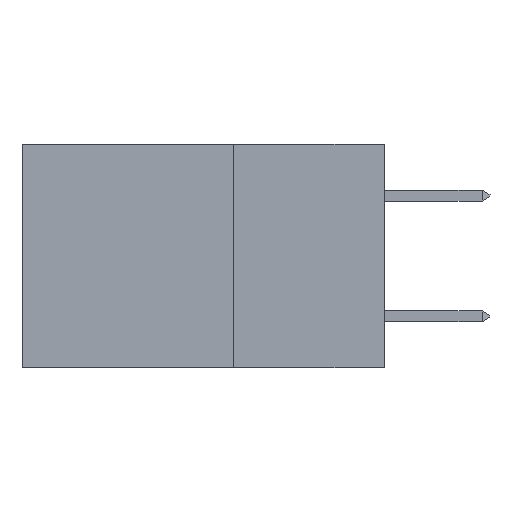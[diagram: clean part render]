
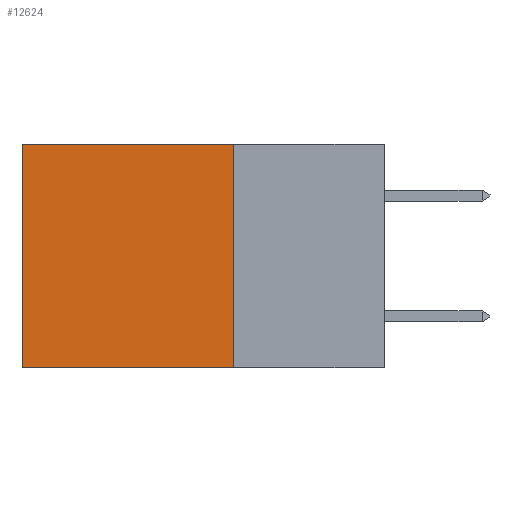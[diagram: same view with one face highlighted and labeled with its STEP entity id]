
A CAD part, left-side view. The second image highlights one B-rep face of the part: STEP entity #12624.
In plain terms, the highlighted planar face has unit normal (-1, 0, 0).
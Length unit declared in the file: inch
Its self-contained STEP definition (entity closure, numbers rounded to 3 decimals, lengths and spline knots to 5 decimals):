
#188 = DIRECTION ( 'NONE',  ( 1., 0., 0. ) ) ;
#495 = LINE ( 'NONE', #3889, #15449 ) ;
#902 = VECTOR ( 'NONE', #17948, 39.37008 ) ;
#945 = EDGE_CURVE ( 'NONE', #18046, #1628, #15442, .T. ) ;
#1114 = VERTEX_POINT ( 'NONE', #2134 ) ;
#1628 = VERTEX_POINT ( 'NONE', #12085 ) ;
#2134 = CARTESIAN_POINT ( 'NONE',  ( 0.2875, 0.6, 0. ) ) ;
#2155 = DIRECTION ( 'NONE',  ( 0., 1., 0. ) ) ;
#3889 = CARTESIAN_POINT ( 'NONE',  ( 0.2875, 0.25, 0. ) ) ;
#4159 = VECTOR ( 'NONE', #2155, 39.37008 ) ;
#5025 = LINE ( 'NONE', #9593, #902 ) ;
#5046 = VECTOR ( 'NONE', #5604, 39.37008 ) ;
#5604 = DIRECTION ( 'NONE',  ( 0., 1., 0. ) ) ;
#6115 = EDGE_LOOP ( 'NONE', ( #16501, #7034, #9757, #9581 ) ) ;
#6490 = CARTESIAN_POINT ( 'NONE',  ( 0.2875, 0.25, -0.37 ) ) ;
#6859 = FACE_OUTER_BOUND ( 'NONE', #6115, .T. ) ;
#6865 = DIRECTION ( 'NONE',  ( 0., 0., -1. ) ) ;
#7034 = ORIENTED_EDGE ( 'NONE', *, *, #945, .F. ) ;
#7261 = VERTEX_POINT ( 'NONE', #15980 ) ;
#9142 = CARTESIAN_POINT ( 'NONE',  ( 0.2875, 0.25, 0. ) ) ;
#9581 = ORIENTED_EDGE ( 'NONE', *, *, #18273, .T. ) ;
#9593 = CARTESIAN_POINT ( 'NONE',  ( 0.2875, 0.6, 0. ) ) ;
#9757 = ORIENTED_EDGE ( 'NONE', *, *, #10001, .F. ) ;
#10001 = EDGE_CURVE ( 'NONE', #7261, #18046, #495, .T. ) ;
#10062 = AXIS2_PLACEMENT_3D ( 'NONE', #9142, #188, #10568 ) ;
#10568 = DIRECTION ( 'NONE',  ( 0., 0., -1. ) ) ;
#12085 = CARTESIAN_POINT ( 'NONE',  ( 0.2875, 0.6, -0.37 ) ) ;
#12173 = EDGE_CURVE ( 'NONE', #1114, #1628, #5025, .T. ) ;
#12624 = ADVANCED_FACE ( 'NONE', ( #6859 ), #17512, .F. ) ;
#15393 = CARTESIAN_POINT ( 'NONE',  ( 0.2875, 0.25, 0. ) ) ;
#15442 = LINE ( 'NONE', #18330, #4159 ) ;
#15449 = VECTOR ( 'NONE', #6865, 39.37008 ) ;
#15980 = CARTESIAN_POINT ( 'NONE',  ( 0.2875, 0.25, 0. ) ) ;
#16501 = ORIENTED_EDGE ( 'NONE', *, *, #12173, .T. ) ;
#17512 = PLANE ( 'NONE',  #10062 ) ;
#17948 = DIRECTION ( 'NONE',  ( 0., 0., -1. ) ) ;
#18046 = VERTEX_POINT ( 'NONE', #6490 ) ;
#18234 = LINE ( 'NONE', #15393, #5046 ) ;
#18273 = EDGE_CURVE ( 'NONE', #7261, #1114, #18234, .T. ) ;
#18330 = CARTESIAN_POINT ( 'NONE',  ( 0.2875, 0.25, -0.37 ) ) ;
